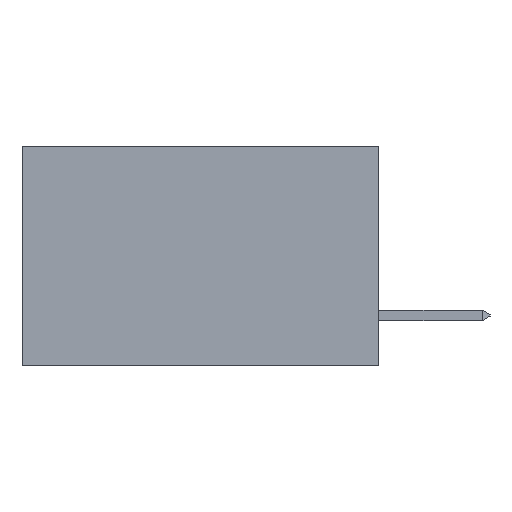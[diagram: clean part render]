
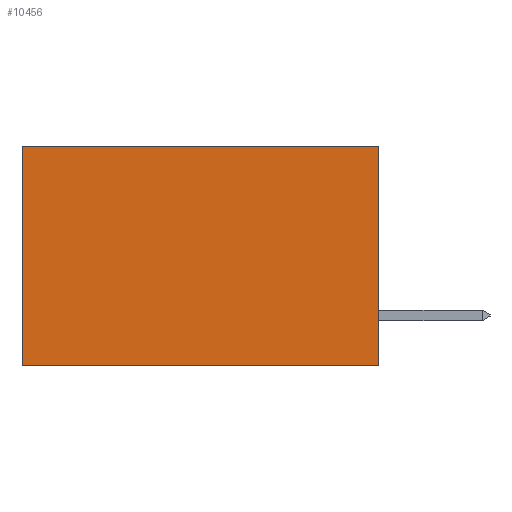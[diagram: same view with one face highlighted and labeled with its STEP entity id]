
A CAD part, left-side view. The second image highlights one B-rep face of the part: STEP entity #10456.
In plain terms, the highlighted planar face has unit normal (-1, 0, 0).
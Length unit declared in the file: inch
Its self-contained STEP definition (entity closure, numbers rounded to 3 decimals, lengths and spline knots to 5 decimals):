
#796 = CARTESIAN_POINT ( 'NONE',  ( 0.298, 0., 0. ) ) ;
#1062 = FACE_OUTER_BOUND ( 'NONE', #1137, .T. ) ;
#1108 = VERTEX_POINT ( 'NONE', #15505 ) ;
#1137 = EDGE_LOOP ( 'NONE', ( #15171, #11377, #15117, #14199 ) ) ;
#2157 = DIRECTION ( 'NONE',  ( 0., 0., -1. ) ) ;
#3552 = EDGE_CURVE ( 'NONE', #1108, #4623, #16212, .T. ) ;
#3665 = CARTESIAN_POINT ( 'NONE',  ( 0.298, 0.6, -0.37 ) ) ;
#4623 = VERTEX_POINT ( 'NONE', #3665 ) ;
#5252 = VERTEX_POINT ( 'NONE', #7350 ) ;
#5649 = CARTESIAN_POINT ( 'NONE',  ( 0.298, 0., 0. ) ) ;
#5794 = VECTOR ( 'NONE', #7315, 39.37008 ) ;
#5980 = CARTESIAN_POINT ( 'NONE',  ( 0.298, 0., -0.37 ) ) ;
#6882 = PLANE ( 'NONE',  #12174 ) ;
#6939 = DIRECTION ( 'NONE',  ( 0., 0., -1. ) ) ;
#7315 = DIRECTION ( 'NONE',  ( 0., 1., 0. ) ) ;
#7350 = CARTESIAN_POINT ( 'NONE',  ( 0.298, 0.6, 0. ) ) ;
#9069 = DIRECTION ( 'NONE',  ( 0., 1., 0. ) ) ;
#9134 = VECTOR ( 'NONE', #13180, 39.37008 ) ;
#9187 = CARTESIAN_POINT ( 'NONE',  ( 0.298, 0., 0. ) ) ;
#9416 = VECTOR ( 'NONE', #2157, 39.37008 ) ;
#9749 = VERTEX_POINT ( 'NONE', #9187 ) ;
#10456 = ADVANCED_FACE ( 'NONE', ( #1062 ), #6882, .F. ) ;
#10662 = CARTESIAN_POINT ( 'NONE',  ( 0.298, 0.6, 0. ) ) ;
#11377 = ORIENTED_EDGE ( 'NONE', *, *, #3552, .F. ) ;
#12174 = AXIS2_PLACEMENT_3D ( 'NONE', #5649, #14701, #6939 ) ;
#12642 = EDGE_CURVE ( 'NONE', #9749, #1108, #13194, .T. ) ;
#12644 = LINE ( 'NONE', #16386, #5794 ) ;
#12927 = LINE ( 'NONE', #10662, #9134 ) ;
#13180 = DIRECTION ( 'NONE',  ( 0., 0., -1. ) ) ;
#13194 = LINE ( 'NONE', #796, #9416 ) ;
#14199 = ORIENTED_EDGE ( 'NONE', *, *, #16205, .T. ) ;
#14701 = DIRECTION ( 'NONE',  ( 1., 0., 0. ) ) ;
#15117 = ORIENTED_EDGE ( 'NONE', *, *, #12642, .F. ) ;
#15171 = ORIENTED_EDGE ( 'NONE', *, *, #15464, .T. ) ;
#15411 = VECTOR ( 'NONE', #9069, 39.37008 ) ;
#15464 = EDGE_CURVE ( 'NONE', #5252, #4623, #12927, .T. ) ;
#15505 = CARTESIAN_POINT ( 'NONE',  ( 0.298, 0., -0.37 ) ) ;
#16205 = EDGE_CURVE ( 'NONE', #9749, #5252, #12644, .T. ) ;
#16212 = LINE ( 'NONE', #5980, #15411 ) ;
#16386 = CARTESIAN_POINT ( 'NONE',  ( 0.298, 0., 0. ) ) ;
